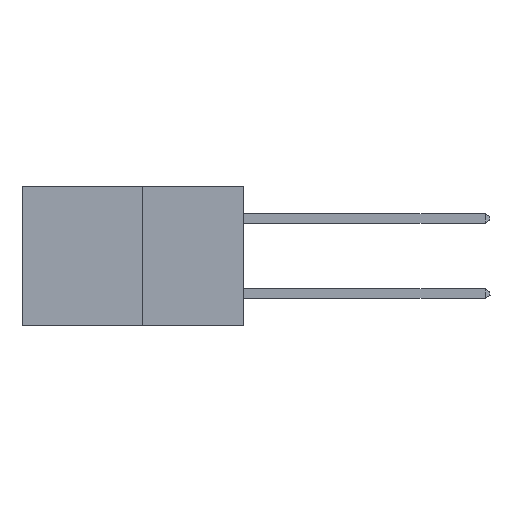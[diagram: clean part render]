
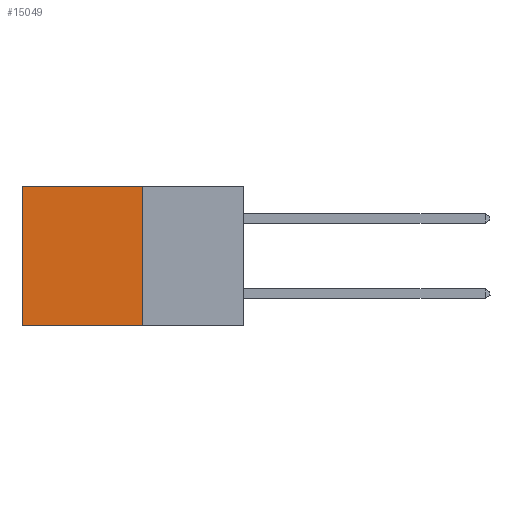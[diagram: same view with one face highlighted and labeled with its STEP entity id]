
A CAD part, left-side view. The second image highlights one B-rep face of the part: STEP entity #15049.
In plain terms, the highlighted planar face has unit normal (-1, 0, 0).
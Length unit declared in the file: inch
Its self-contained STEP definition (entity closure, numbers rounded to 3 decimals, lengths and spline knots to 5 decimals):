
#351 = LINE ( 'NONE', #16408, #3475 ) ;
#490 = LINE ( 'NONE', #3582, #10813 ) ;
#1809 = LINE ( 'NONE', #14568, #16021 ) ;
#2095 = VERTEX_POINT ( 'NONE', #13258 ) ;
#3475 = VECTOR ( 'NONE', #11172, 39.37008 ) ;
#3582 = CARTESIAN_POINT ( 'NONE',  ( 0.277, 0.27, -0.37 ) ) ;
#4921 = DIRECTION ( 'NONE',  ( 0., 1., 0. ) ) ;
#5030 = VERTEX_POINT ( 'NONE', #5044 ) ;
#5044 = CARTESIAN_POINT ( 'NONE',  ( 0.277, 0.59, 0. ) ) ;
#5131 = DIRECTION ( 'NONE',  ( 1., 0., 0. ) ) ;
#5181 = CARTESIAN_POINT ( 'NONE',  ( 0.277, 0.27, -0.37 ) ) ;
#6010 = EDGE_LOOP ( 'NONE', ( #10851, #7860, #11943, #13974 ) ) ;
#6460 = VERTEX_POINT ( 'NONE', #8052 ) ;
#6540 = VERTEX_POINT ( 'NONE', #14439 ) ;
#6548 = PLANE ( 'NONE',  #13663 ) ;
#7802 = LINE ( 'NONE', #9782, #14440 ) ;
#7860 = ORIENTED_EDGE ( 'NONE', *, *, #13011, .F. ) ;
#7937 = DIRECTION ( 'NONE',  ( 0., 0., -1. ) ) ;
#8052 = CARTESIAN_POINT ( 'NONE',  ( 0.277, 0.27, 0. ) ) ;
#8538 = FACE_OUTER_BOUND ( 'NONE', #6010, .T. ) ;
#8755 = EDGE_CURVE ( 'NONE', #6460, #5030, #7802, .T. ) ;
#9550 = EDGE_CURVE ( 'NONE', #6460, #6540, #1809, .T. ) ;
#9782 = CARTESIAN_POINT ( 'NONE',  ( 0.277, 0.27, 0. ) ) ;
#10813 = VECTOR ( 'NONE', #4921, 39.37008 ) ;
#10851 = ORIENTED_EDGE ( 'NONE', *, *, #11460, .T. ) ;
#11172 = DIRECTION ( 'NONE',  ( 0., 0., -1. ) ) ;
#11460 = EDGE_CURVE ( 'NONE', #5030, #2095, #351, .T. ) ;
#11943 = ORIENTED_EDGE ( 'NONE', *, *, #9550, .F. ) ;
#13011 = EDGE_CURVE ( 'NONE', #6540, #2095, #490, .T. ) ;
#13258 = CARTESIAN_POINT ( 'NONE',  ( 0.277, 0.59, -0.37 ) ) ;
#13663 = AXIS2_PLACEMENT_3D ( 'NONE', #5181, #5131, #7937 ) ;
#13974 = ORIENTED_EDGE ( 'NONE', *, *, #8755, .T. ) ;
#14175 = DIRECTION ( 'NONE',  ( 0., 1., 0. ) ) ;
#14439 = CARTESIAN_POINT ( 'NONE',  ( 0.277, 0.27, -0.37 ) ) ;
#14440 = VECTOR ( 'NONE', #14175, 39.37008 ) ;
#14568 = CARTESIAN_POINT ( 'NONE',  ( 0.277, 0.27, -0.37 ) ) ;
#14787 = DIRECTION ( 'NONE',  ( 0., 0., -1. ) ) ;
#15049 = ADVANCED_FACE ( 'NONE', ( #8538 ), #6548, .F. ) ;
#16021 = VECTOR ( 'NONE', #14787, 39.37008 ) ;
#16408 = CARTESIAN_POINT ( 'NONE',  ( 0.277, 0.59, -0.37 ) ) ;
